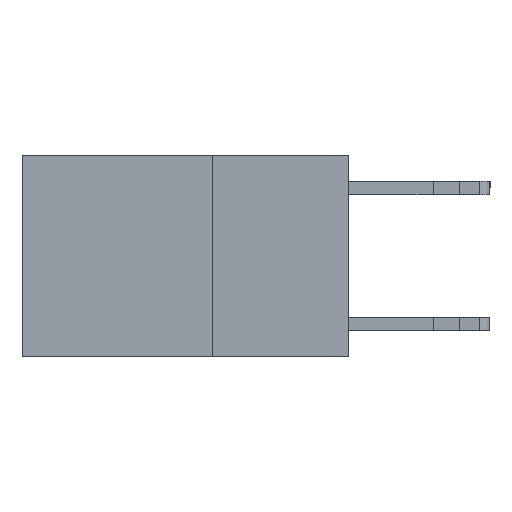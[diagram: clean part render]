
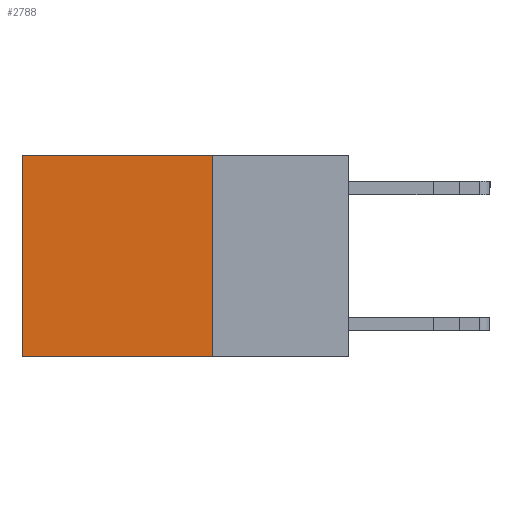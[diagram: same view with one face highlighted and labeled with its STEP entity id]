
A CAD part, left-side view. The second image highlights one B-rep face of the part: STEP entity #2788.
In plain terms, the highlighted planar face has unit normal (-1, 0, 0).
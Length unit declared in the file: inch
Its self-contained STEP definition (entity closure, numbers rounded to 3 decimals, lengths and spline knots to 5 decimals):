
#47 = ORIENTED_EDGE ( 'NONE', *, *, #11507, .F. ) ;
#283 = VECTOR ( 'NONE', #12060, 39.37008 ) ;
#539 = LINE ( 'NONE', #15009, #13682 ) ;
#625 = DIRECTION ( 'NONE',  ( 0., 0., -1. ) ) ;
#2595 = ORIENTED_EDGE ( 'NONE', *, *, #11603, .T. ) ;
#2692 = CARTESIAN_POINT ( 'NONE',  ( 0.2625, 0.25, 0. ) ) ;
#2744 = EDGE_CURVE ( 'NONE', #10222, #9276, #539, .T. ) ;
#2788 = ADVANCED_FACE ( 'NONE', ( #5818 ), #8288, .F. ) ;
#2814 = LINE ( 'NONE', #8037, #10185 ) ;
#3410 = DIRECTION ( 'NONE',  ( 0., 1., 0. ) ) ;
#4351 = DIRECTION ( 'NONE',  ( 0., 1., 0. ) ) ;
#5726 = VERTEX_POINT ( 'NONE', #6201 ) ;
#5818 = FACE_OUTER_BOUND ( 'NONE', #16051, .T. ) ;
#6201 = CARTESIAN_POINT ( 'NONE',  ( 0.2625, 0.25, -0.37 ) ) ;
#6759 = EDGE_CURVE ( 'NONE', #10222, #5726, #8005, .T. ) ;
#6943 = CARTESIAN_POINT ( 'NONE',  ( 0.2625, 0.25, -0.37 ) ) ;
#7624 = CARTESIAN_POINT ( 'NONE',  ( 0.2625, 0.25, 0. ) ) ;
#8005 = LINE ( 'NONE', #2692, #283 ) ;
#8037 = CARTESIAN_POINT ( 'NONE',  ( 0.2625, 0.6, 0. ) ) ;
#8288 = PLANE ( 'NONE',  #13768 ) ;
#9276 = VERTEX_POINT ( 'NONE', #16463 ) ;
#10185 = VECTOR ( 'NONE', #10556, 39.37008 ) ;
#10222 = VERTEX_POINT ( 'NONE', #7624 ) ;
#10556 = DIRECTION ( 'NONE',  ( 0., 0., -1. ) ) ;
#11287 = VERTEX_POINT ( 'NONE', #15026 ) ;
#11507 = EDGE_CURVE ( 'NONE', #5726, #11287, #13219, .T. ) ;
#11603 = EDGE_CURVE ( 'NONE', #9276, #11287, #2814, .T. ) ;
#12060 = DIRECTION ( 'NONE',  ( 0., 0., -1. ) ) ;
#12636 = VECTOR ( 'NONE', #4351, 39.37008 ) ;
#13219 = LINE ( 'NONE', #6943, #12636 ) ;
#13682 = VECTOR ( 'NONE', #3410, 39.37008 ) ;
#13768 = AXIS2_PLACEMENT_3D ( 'NONE', #15175, #14841, #625 ) ;
#14841 = DIRECTION ( 'NONE',  ( 1., 0., 0. ) ) ;
#15009 = CARTESIAN_POINT ( 'NONE',  ( 0.2625, 0.25, 0. ) ) ;
#15026 = CARTESIAN_POINT ( 'NONE',  ( 0.2625, 0.6, -0.37 ) ) ;
#15119 = ORIENTED_EDGE ( 'NONE', *, *, #2744, .T. ) ;
#15175 = CARTESIAN_POINT ( 'NONE',  ( 0.2625, 0.25, 0. ) ) ;
#16051 = EDGE_LOOP ( 'NONE', ( #2595, #47, #16353, #15119 ) ) ;
#16353 = ORIENTED_EDGE ( 'NONE', *, *, #6759, .F. ) ;
#16463 = CARTESIAN_POINT ( 'NONE',  ( 0.2625, 0.6, 0. ) ) ;
